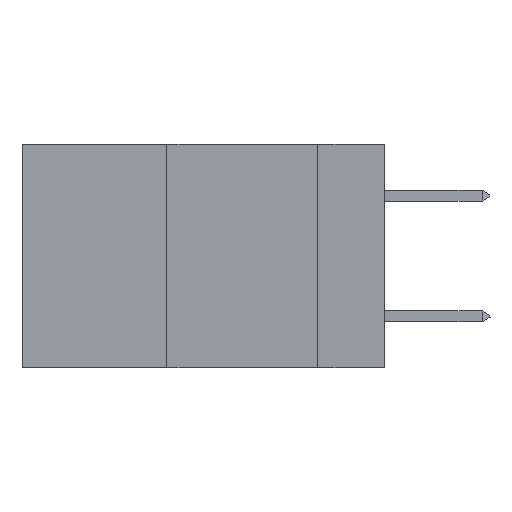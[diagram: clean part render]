
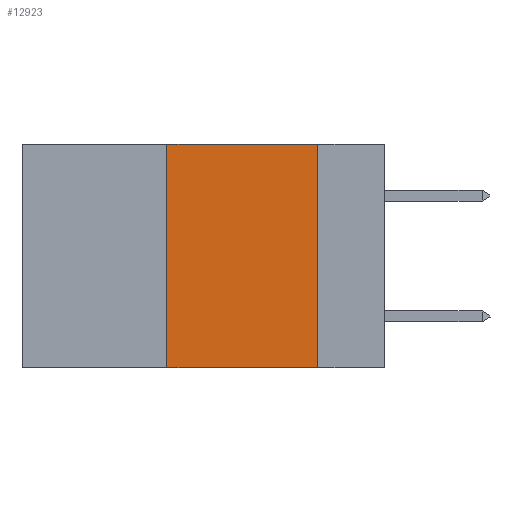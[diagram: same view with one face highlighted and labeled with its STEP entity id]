
A CAD part, left-side view. The second image highlights one B-rep face of the part: STEP entity #12923.
In plain terms, the highlighted planar face has unit normal (-1, 0, 0).
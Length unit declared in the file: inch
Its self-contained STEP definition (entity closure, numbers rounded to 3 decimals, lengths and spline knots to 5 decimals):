
#67 = EDGE_CURVE ( 'NONE', #4937, #13145, #6903, .T. ) ;
#889 = ORIENTED_EDGE ( 'NONE', *, *, #67, .T. ) ;
#1251 = LINE ( 'NONE', #12042, #15516 ) ;
#1605 = CARTESIAN_POINT ( 'NONE',  ( 0., 0.6, -0.37 ) ) ;
#1733 = VECTOR ( 'NONE', #15314, 39.37008 ) ;
#1752 = DIRECTION ( 'NONE',  ( 0., 0., -1. ) ) ;
#1754 = LINE ( 'NONE', #4882, #2617 ) ;
#2617 = VECTOR ( 'NONE', #3289, 39.37008 ) ;
#3289 = DIRECTION ( 'NONE',  ( 0., 0., -1. ) ) ;
#4101 = EDGE_CURVE ( 'NONE', #8908, #8702, #16550, .T. ) ;
#4882 = CARTESIAN_POINT ( 'NONE',  ( 0., 0.11, 0. ) ) ;
#4937 = VERTEX_POINT ( 'NONE', #10131 ) ;
#5795 = CARTESIAN_POINT ( 'NONE',  ( 0., 0.6, 0. ) ) ;
#5827 = CARTESIAN_POINT ( 'NONE',  ( 0., 0.6, 0. ) ) ;
#6747 = FACE_OUTER_BOUND ( 'NONE', #10816, .T. ) ;
#6903 = LINE ( 'NONE', #1605, #1733 ) ;
#7206 = EDGE_CURVE ( 'NONE', #8702, #13145, #1754, .T. ) ;
#7330 = DIRECTION ( 'NONE',  ( 0., -1., 0. ) ) ;
#8702 = VERTEX_POINT ( 'NONE', #9762 ) ;
#8734 = PLANE ( 'NONE',  #13804 ) ;
#8908 = VERTEX_POINT ( 'NONE', #13315 ) ;
#9762 = CARTESIAN_POINT ( 'NONE',  ( 0., 0.11, 0. ) ) ;
#10131 = CARTESIAN_POINT ( 'NONE',  ( 0., 0.36, -0.37 ) ) ;
#10816 = EDGE_LOOP ( 'NONE', ( #11020, #11893, #13381, #889 ) ) ;
#11020 = ORIENTED_EDGE ( 'NONE', *, *, #7206, .F. ) ;
#11893 = ORIENTED_EDGE ( 'NONE', *, *, #4101, .F. ) ;
#12042 = CARTESIAN_POINT ( 'NONE',  ( 0., 0.36, 0. ) ) ;
#12411 = CARTESIAN_POINT ( 'NONE',  ( 0., 0.11, -0.37 ) ) ;
#12923 = ADVANCED_FACE ( 'NONE', ( #6747 ), #8734, .F. ) ;
#13145 = VERTEX_POINT ( 'NONE', #12411 ) ;
#13315 = CARTESIAN_POINT ( 'NONE',  ( 0., 0.36, 0. ) ) ;
#13381 = ORIENTED_EDGE ( 'NONE', *, *, #17305, .F. ) ;
#13804 = AXIS2_PLACEMENT_3D ( 'NONE', #5827, #15343, #1752 ) ;
#14446 = VECTOR ( 'NONE', #7330, 39.37008 ) ;
#15314 = DIRECTION ( 'NONE',  ( 0., -1., 0. ) ) ;
#15343 = DIRECTION ( 'NONE',  ( 1., 0., 0. ) ) ;
#15516 = VECTOR ( 'NONE', #16095, 39.37008 ) ;
#16095 = DIRECTION ( 'NONE',  ( 0., 0., 1. ) ) ;
#16550 = LINE ( 'NONE', #5795, #14446 ) ;
#17305 = EDGE_CURVE ( 'NONE', #4937, #8908, #1251, .T. ) ;
